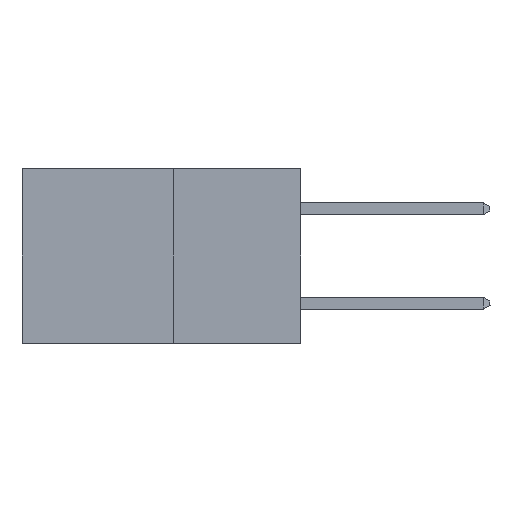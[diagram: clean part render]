
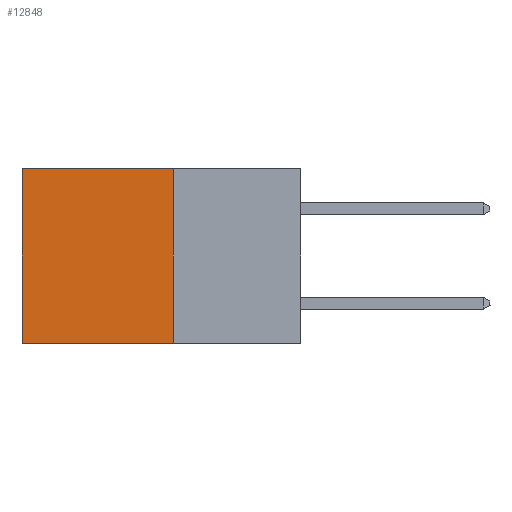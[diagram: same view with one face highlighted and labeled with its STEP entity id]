
A CAD part, left-side view. The second image highlights one B-rep face of the part: STEP entity #12848.
In plain terms, the highlighted planar face has unit normal (-1, 0, 0).
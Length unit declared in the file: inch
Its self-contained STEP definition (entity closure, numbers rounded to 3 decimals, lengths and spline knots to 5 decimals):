
#689 = VECTOR ( 'NONE', #10188, 39.37008 ) ;
#944 = ORIENTED_EDGE ( 'NONE', *, *, #12253, .T. ) ;
#1006 = ORIENTED_EDGE ( 'NONE', *, *, #11566, .F. ) ;
#1522 = ORIENTED_EDGE ( 'NONE', *, *, #6364, .F. ) ;
#1690 = ORIENTED_EDGE ( 'NONE', *, *, #4468, .T. ) ;
#1785 = VERTEX_POINT ( 'NONE', #2397 ) ;
#2397 = CARTESIAN_POINT ( 'NONE',  ( 0.277, 0.27, -0.37 ) ) ;
#3755 = CARTESIAN_POINT ( 'NONE',  ( 0.277, 0.27, -0.37 ) ) ;
#3986 = CARTESIAN_POINT ( 'NONE',  ( 0.277, 0.59, -0.37 ) ) ;
#4468 = EDGE_CURVE ( 'NONE', #12722, #5049, #7651, .T. ) ;
#4659 = VERTEX_POINT ( 'NONE', #13892 ) ;
#5043 = DIRECTION ( 'NONE',  ( 1., 0., 0. ) ) ;
#5049 = VERTEX_POINT ( 'NONE', #5145 ) ;
#5145 = CARTESIAN_POINT ( 'NONE',  ( 0.277, 0.59, 0. ) ) ;
#5301 = CARTESIAN_POINT ( 'NONE',  ( 0.277, 0.27, -0.37 ) ) ;
#6364 = EDGE_CURVE ( 'NONE', #12722, #1785, #8734, .T. ) ;
#6668 = VECTOR ( 'NONE', #12398, 39.37008 ) ;
#7341 = CARTESIAN_POINT ( 'NONE',  ( 0.277, 0.27, -0.37 ) ) ;
#7544 = AXIS2_PLACEMENT_3D ( 'NONE', #3755, #5043, #13296 ) ;
#7651 = LINE ( 'NONE', #15586, #689 ) ;
#7948 = DIRECTION ( 'NONE',  ( 0., 0., -1. ) ) ;
#8679 = EDGE_LOOP ( 'NONE', ( #944, #1006, #1522, #1690 ) ) ;
#8734 = LINE ( 'NONE', #7341, #11777 ) ;
#9682 = CARTESIAN_POINT ( 'NONE',  ( 0.277, 0.27, 0. ) ) ;
#9968 = VECTOR ( 'NONE', #12382, 39.37008 ) ;
#10188 = DIRECTION ( 'NONE',  ( 0., 1., 0. ) ) ;
#11027 = PLANE ( 'NONE',  #7544 ) ;
#11566 = EDGE_CURVE ( 'NONE', #1785, #4659, #12491, .T. ) ;
#11777 = VECTOR ( 'NONE', #7948, 39.37008 ) ;
#12253 = EDGE_CURVE ( 'NONE', #5049, #4659, #15262, .T. ) ;
#12382 = DIRECTION ( 'NONE',  ( 0., 0., -1. ) ) ;
#12398 = DIRECTION ( 'NONE',  ( 0., 1., 0. ) ) ;
#12491 = LINE ( 'NONE', #5301, #6668 ) ;
#12722 = VERTEX_POINT ( 'NONE', #9682 ) ;
#12848 = ADVANCED_FACE ( 'NONE', ( #13853 ), #11027, .F. ) ;
#13296 = DIRECTION ( 'NONE',  ( 0., 0., -1. ) ) ;
#13853 = FACE_OUTER_BOUND ( 'NONE', #8679, .T. ) ;
#13892 = CARTESIAN_POINT ( 'NONE',  ( 0.277, 0.59, -0.37 ) ) ;
#15262 = LINE ( 'NONE', #3986, #9968 ) ;
#15586 = CARTESIAN_POINT ( 'NONE',  ( 0.277, 0.27, 0. ) ) ;
